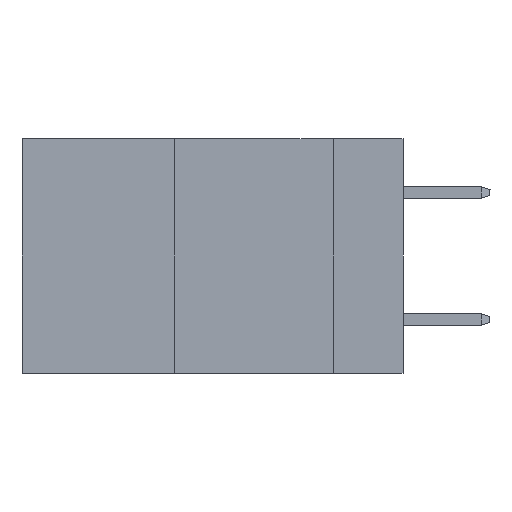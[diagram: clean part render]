
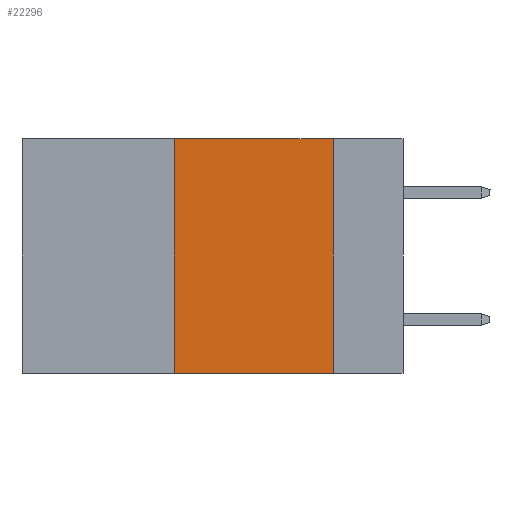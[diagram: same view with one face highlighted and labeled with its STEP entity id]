
A CAD part, left-side view. The second image highlights one B-rep face of the part: STEP entity #22296.
In plain terms, the highlighted planar face has unit normal (-1, 0, 0).
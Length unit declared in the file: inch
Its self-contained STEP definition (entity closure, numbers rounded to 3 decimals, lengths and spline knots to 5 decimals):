
#3138 = VERTEX_POINT ( 'NONE', #20109 ) ;
#3492 = DIRECTION ( 'NONE',  ( 0., 0., -1. ) ) ;
#3668 = DIRECTION ( 'NONE',  ( 0., 0., 1. ) ) ;
#4155 = DIRECTION ( 'NONE',  ( 0., -1., 0. ) ) ;
#4185 = EDGE_LOOP ( 'NONE', ( #13615, #8310, #9007, #25809 ) ) ;
#4900 = VERTEX_POINT ( 'NONE', #25315 ) ;
#4931 = EDGE_CURVE ( 'NONE', #25254, #20258, #17142, .T. ) ;
#6301 = LINE ( 'NONE', #15164, #21352 ) ;
#7102 = AXIS2_PLACEMENT_3D ( 'NONE', #20369, #32228, #3492 ) ;
#7801 = VECTOR ( 'NONE', #17337, 39.37008 ) ;
#8310 = ORIENTED_EDGE ( 'NONE', *, *, #17005, .F. ) ;
#9007 = ORIENTED_EDGE ( 'NONE', *, *, #31877, .F. ) ;
#9450 = CARTESIAN_POINT ( 'NONE',  ( 0., 0.36, 0. ) ) ;
#11415 = FACE_OUTER_BOUND ( 'NONE', #4185, .T. ) ;
#13615 = ORIENTED_EDGE ( 'NONE', *, *, #28150, .F. ) ;
#14294 = CARTESIAN_POINT ( 'NONE',  ( 0., 0.36, -0.37 ) ) ;
#15164 = CARTESIAN_POINT ( 'NONE',  ( 0., 0.6, 0. ) ) ;
#17005 = EDGE_CURVE ( 'NONE', #3138, #4900, #6301, .T. ) ;
#17142 = LINE ( 'NONE', #29003, #7801 ) ;
#17337 = DIRECTION ( 'NONE',  ( 0., -1., 0. ) ) ;
#19421 = VECTOR ( 'NONE', #22582, 39.37008 ) ;
#20109 = CARTESIAN_POINT ( 'NONE',  ( 0., 0.36, 0. ) ) ;
#20258 = VERTEX_POINT ( 'NONE', #25135 ) ;
#20369 = CARTESIAN_POINT ( 'NONE',  ( 0., 0.6, 0. ) ) ;
#21352 = VECTOR ( 'NONE', #4155, 39.37008 ) ;
#22296 = ADVANCED_FACE ( 'NONE', ( #11415 ), #23256, .F. ) ;
#22582 = DIRECTION ( 'NONE',  ( 0., 0., -1. ) ) ;
#23256 = PLANE ( 'NONE',  #7102 ) ;
#23695 = VECTOR ( 'NONE', #3668, 39.37008 ) ;
#25135 = CARTESIAN_POINT ( 'NONE',  ( 0., 0.11, -0.37 ) ) ;
#25254 = VERTEX_POINT ( 'NONE', #14294 ) ;
#25315 = CARTESIAN_POINT ( 'NONE',  ( 0., 0.11, 0. ) ) ;
#25809 = ORIENTED_EDGE ( 'NONE', *, *, #4931, .T. ) ;
#26741 = LINE ( 'NONE', #9450, #23695 ) ;
#28150 = EDGE_CURVE ( 'NONE', #4900, #20258, #32128, .T. ) ;
#29003 = CARTESIAN_POINT ( 'NONE',  ( 0., 0.6, -0.37 ) ) ;
#31877 = EDGE_CURVE ( 'NONE', #25254, #3138, #26741, .T. ) ;
#31936 = CARTESIAN_POINT ( 'NONE',  ( 0., 0.11, 0. ) ) ;
#32128 = LINE ( 'NONE', #31936, #19421 ) ;
#32228 = DIRECTION ( 'NONE',  ( 1., 0., 0. ) ) ;
